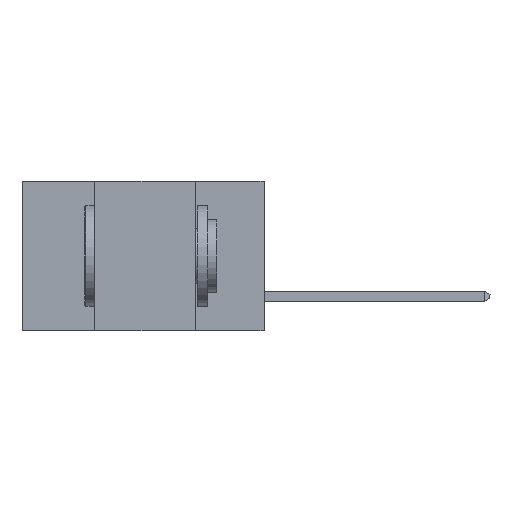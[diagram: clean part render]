
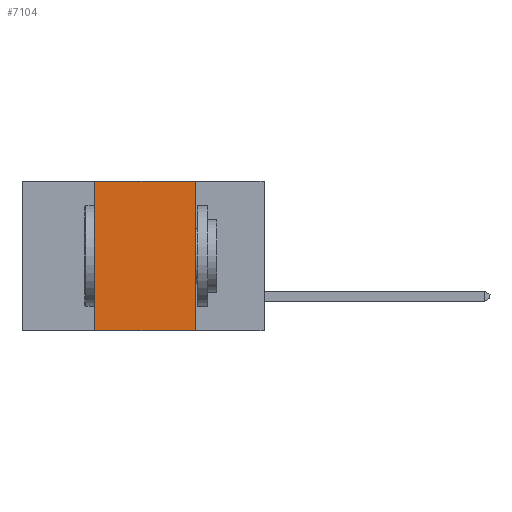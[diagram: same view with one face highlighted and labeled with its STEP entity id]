
A CAD part, left-side view. The second image highlights one B-rep face of the part: STEP entity #7104.
In plain terms, the highlighted planar face has unit normal (-1, 0, 0).
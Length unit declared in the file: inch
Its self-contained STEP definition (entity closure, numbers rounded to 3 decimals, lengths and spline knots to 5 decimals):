
#184 = AXIS2_PLACEMENT_3D ( 'NONE', #5403, #7074, #1513 ) ;
#710 = VERTEX_POINT ( 'NONE', #7103 ) ;
#798 = DIRECTION ( 'NONE',  ( 0., -1., 0. ) ) ;
#982 = EDGE_CURVE ( 'NONE', #710, #6861, #2890, .T. ) ;
#1087 = ORIENTED_EDGE ( 'NONE', *, *, #3474, .F. ) ;
#1454 = DIRECTION ( 'NONE',  ( 0., -1., 0. ) ) ;
#1513 = DIRECTION ( 'NONE',  ( 0., 0., -1. ) ) ;
#1673 = LINE ( 'NONE', #5676, #2729 ) ;
#2347 = ORIENTED_EDGE ( 'NONE', *, *, #7448, .T. ) ;
#2628 = CARTESIAN_POINT ( 'NONE',  ( 0., 0.17, 0. ) ) ;
#2689 = CARTESIAN_POINT ( 'NONE',  ( 0., 0.42, -0.37 ) ) ;
#2729 = VECTOR ( 'NONE', #1454, 39.37008 ) ;
#2890 = LINE ( 'NONE', #2689, #3371 ) ;
#3074 = DIRECTION ( 'NONE',  ( 0., 0., -1. ) ) ;
#3371 = VECTOR ( 'NONE', #8416, 39.37008 ) ;
#3474 = EDGE_CURVE ( 'NONE', #5807, #7021, #3977, .T. ) ;
#3897 = CARTESIAN_POINT ( 'NONE',  ( 0., 0.6, -0.37 ) ) ;
#3977 = LINE ( 'NONE', #10415, #7293 ) ;
#4261 = VECTOR ( 'NONE', #798, 39.37008 ) ;
#5299 = EDGE_CURVE ( 'NONE', #6861, #5807, #1673, .T. ) ;
#5403 = CARTESIAN_POINT ( 'NONE',  ( 0., 0.6, 0. ) ) ;
#5572 = PLANE ( 'NONE',  #184 ) ;
#5676 = CARTESIAN_POINT ( 'NONE',  ( 0., 0.6, 0. ) ) ;
#5807 = VERTEX_POINT ( 'NONE', #2628 ) ;
#6861 = VERTEX_POINT ( 'NONE', #8429 ) ;
#7021 = VERTEX_POINT ( 'NONE', #7817 ) ;
#7074 = DIRECTION ( 'NONE',  ( 1., 0., 0. ) ) ;
#7103 = CARTESIAN_POINT ( 'NONE',  ( 0., 0.42, -0.37 ) ) ;
#7104 = ADVANCED_FACE ( 'NONE', ( #8847 ), #5572, .F. ) ;
#7293 = VECTOR ( 'NONE', #3074, 39.37008 ) ;
#7448 = EDGE_CURVE ( 'NONE', #710, #7021, #9581, .T. ) ;
#7519 = ORIENTED_EDGE ( 'NONE', *, *, #982, .F. ) ;
#7559 = ORIENTED_EDGE ( 'NONE', *, *, #5299, .F. ) ;
#7817 = CARTESIAN_POINT ( 'NONE',  ( 0., 0.17, -0.37 ) ) ;
#8416 = DIRECTION ( 'NONE',  ( 0., 0., 1. ) ) ;
#8429 = CARTESIAN_POINT ( 'NONE',  ( 0., 0.42, 0. ) ) ;
#8847 = FACE_OUTER_BOUND ( 'NONE', #9867, .T. ) ;
#9581 = LINE ( 'NONE', #3897, #4261 ) ;
#9867 = EDGE_LOOP ( 'NONE', ( #1087, #7559, #7519, #2347 ) ) ;
#10415 = CARTESIAN_POINT ( 'NONE',  ( 0., 0.17, -0.37 ) ) ;
